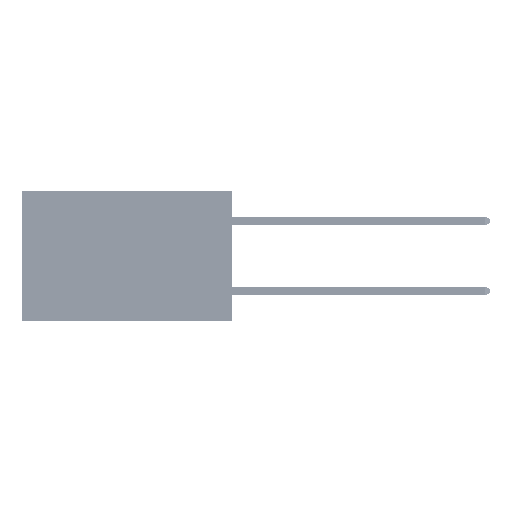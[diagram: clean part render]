
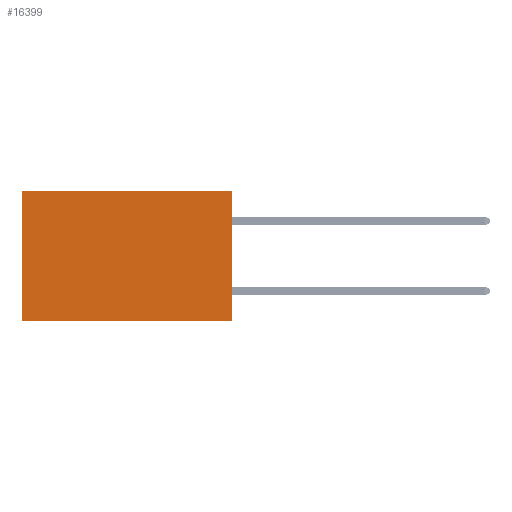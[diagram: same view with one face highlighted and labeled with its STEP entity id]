
A CAD part, left-side view. The second image highlights one B-rep face of the part: STEP entity #16399.
In plain terms, the highlighted planar face has unit normal (-1, 0, 0).
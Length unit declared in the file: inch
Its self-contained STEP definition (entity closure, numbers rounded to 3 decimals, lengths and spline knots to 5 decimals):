
#98 = LINE ( 'NONE', #6280, #7631 ) ;
#168 = VECTOR ( 'NONE', #43000, 39.37008 ) ;
#1747 = LINE ( 'NONE', #45806, #7384 ) ;
#2336 = DIRECTION ( 'NONE',  ( 0., 1., 0. ) ) ;
#5289 = DIRECTION ( 'NONE',  ( 0., 1., 0. ) ) ;
#5301 = LINE ( 'NONE', #46032, #39221 ) ;
#6280 = CARTESIAN_POINT ( 'NONE',  ( 0.2875, 0., 0. ) ) ;
#7384 = VECTOR ( 'NONE', #5289, 39.37008 ) ;
#7631 = VECTOR ( 'NONE', #26298, 39.37008 ) ;
#9902 = PLANE ( 'NONE',  #24734 ) ;
#10546 = EDGE_CURVE ( 'NONE', #31309, #33206, #5301, .T. ) ;
#10604 = DIRECTION ( 'NONE',  ( 1., 0., 0. ) ) ;
#13115 = EDGE_CURVE ( 'NONE', #31309, #31313, #98, .T. ) ;
#16399 = ADVANCED_FACE ( 'NONE', ( #33171 ), #9902, .F. ) ;
#16931 = CARTESIAN_POINT ( 'NONE',  ( 0.2875, 0., 0. ) ) ;
#18524 = DIRECTION ( 'NONE',  ( 0., 0., -1. ) ) ;
#18713 = ORIENTED_EDGE ( 'NONE', *, *, #26593, .T. ) ;
#22869 = CARTESIAN_POINT ( 'NONE',  ( 0.2875, 0.6, 0. ) ) ;
#24734 = AXIS2_PLACEMENT_3D ( 'NONE', #26202, #10604, #18524 ) ;
#25128 = CARTESIAN_POINT ( 'NONE',  ( 0.2875, 0.6, 0. ) ) ;
#25143 = CARTESIAN_POINT ( 'NONE',  ( 0.2875, 0., -0.37 ) ) ;
#26202 = CARTESIAN_POINT ( 'NONE',  ( 0.2875, 0., 0. ) ) ;
#26298 = DIRECTION ( 'NONE',  ( 0., 0., -1. ) ) ;
#26593 = EDGE_CURVE ( 'NONE', #33206, #45408, #49795, .T. ) ;
#27878 = ORIENTED_EDGE ( 'NONE', *, *, #10546, .T. ) ;
#31087 = ORIENTED_EDGE ( 'NONE', *, *, #13115, .F. ) ;
#31309 = VERTEX_POINT ( 'NONE', #16931 ) ;
#31313 = VERTEX_POINT ( 'NONE', #25143 ) ;
#31452 = EDGE_CURVE ( 'NONE', #31313, #45408, #1747, .T. ) ;
#33171 = FACE_OUTER_BOUND ( 'NONE', #41183, .T. ) ;
#33206 = VERTEX_POINT ( 'NONE', #25128 ) ;
#35037 = CARTESIAN_POINT ( 'NONE',  ( 0.2875, 0.6, -0.37 ) ) ;
#39221 = VECTOR ( 'NONE', #2336, 39.37008 ) ;
#41183 = EDGE_LOOP ( 'NONE', ( #18713, #41428, #31087, #27878 ) ) ;
#41428 = ORIENTED_EDGE ( 'NONE', *, *, #31452, .F. ) ;
#43000 = DIRECTION ( 'NONE',  ( 0., 0., -1. ) ) ;
#45408 = VERTEX_POINT ( 'NONE', #35037 ) ;
#45806 = CARTESIAN_POINT ( 'NONE',  ( 0.2875, 0., -0.37 ) ) ;
#46032 = CARTESIAN_POINT ( 'NONE',  ( 0.2875, 0., 0. ) ) ;
#49795 = LINE ( 'NONE', #22869, #168 ) ;
